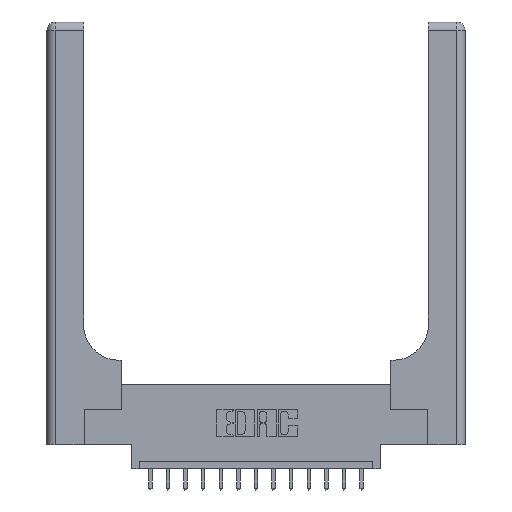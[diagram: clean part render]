
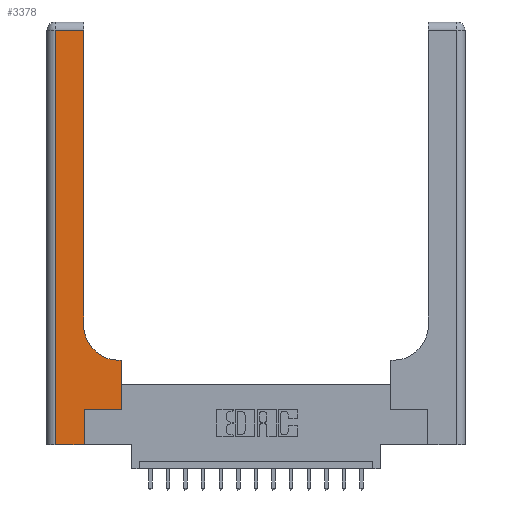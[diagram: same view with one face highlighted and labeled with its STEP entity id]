
A CAD part, top view. The second image highlights one B-rep face of the part: STEP entity #3378.
In plain terms, the highlighted planar face has unit normal (0, 0, 1).
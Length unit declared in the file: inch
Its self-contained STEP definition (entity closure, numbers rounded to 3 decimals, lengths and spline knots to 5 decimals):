
#243 = VECTOR ( 'NONE', #7888, 39.37008 ) ;
#748 = LINE ( 'NONE', #6214, #14005 ) ;
#1354 = VECTOR ( 'NONE', #13960, 39.37008 ) ;
#1579 = PLANE ( 'NONE',  #6849 ) ;
#1590 = VERTEX_POINT ( 'NONE', #4642 ) ;
#1619 = VERTEX_POINT ( 'NONE', #2319 ) ;
#1868 = LINE ( 'NONE', #14319, #16953 ) ;
#1898 = CARTESIAN_POINT ( 'NONE',  ( 0.26, 3., 0.37 ) ) ;
#1962 = CARTESIAN_POINT ( 'NONE',  ( 0.528, 0.6, 0.37 ) ) ;
#2051 = CARTESIAN_POINT ( 'NONE',  ( 0.51, 0.6, 0.37 ) ) ;
#2319 = CARTESIAN_POINT ( 'NONE',  ( 0.528, 0.25, 0.37 ) ) ;
#2332 = ORIENTED_EDGE ( 'NONE', *, *, #17674, .T. ) ;
#2398 = EDGE_CURVE ( 'NONE', #16192, #16802, #6382, .T. ) ;
#2565 = LINE ( 'NONE', #15019, #3959 ) ;
#2573 = DIRECTION ( 'NONE',  ( 1., 0., 0. ) ) ;
#2985 = FACE_OUTER_BOUND ( 'NONE', #3312, .T. ) ;
#3312 = EDGE_LOOP ( 'NONE', ( #5501, #2332, #15300, #16200, #12542, #15239, #9131, #7855, #4134 ) ) ;
#3378 = ADVANCED_FACE ( 'NONE', ( #2985 ), #1579, .F. ) ;
#3959 = VECTOR ( 'NONE', #7848, 39.37008 ) ;
#4134 = ORIENTED_EDGE ( 'NONE', *, *, #4940, .T. ) ;
#4642 = CARTESIAN_POINT ( 'NONE',  ( 0.265, 0., 0.37 ) ) ;
#4940 = EDGE_CURVE ( 'NONE', #8754, #14505, #15435, .T. ) ;
#5501 = ORIENTED_EDGE ( 'NONE', *, *, #15039, .T. ) ;
#6214 = CARTESIAN_POINT ( 'NONE',  ( 0.265, 0.25, 0.37 ) ) ;
#6382 = LINE ( 'NONE', #8626, #243 ) ;
#6792 = CARTESIAN_POINT ( 'NONE',  ( 0.265, 0., 0.37 ) ) ;
#6849 = AXIS2_PLACEMENT_3D ( 'NONE', #14032, #7024, #11344 ) ;
#7024 = DIRECTION ( 'NONE',  ( 0., 0., -1. ) ) ;
#7733 = EDGE_CURVE ( 'NONE', #1619, #10511, #1868, .T. ) ;
#7848 = DIRECTION ( 'NONE',  ( -1., 0., 0. ) ) ;
#7855 = ORIENTED_EDGE ( 'NONE', *, *, #15925, .T. ) ;
#7888 = DIRECTION ( 'NONE',  ( 0., -1., 0. ) ) ;
#8217 = LINE ( 'NONE', #6792, #14340 ) ;
#8593 = VERTEX_POINT ( 'NONE', #10512 ) ;
#8626 = CARTESIAN_POINT ( 'NONE',  ( 0.06, 3., 0.37 ) ) ;
#8656 = CARTESIAN_POINT ( 'NONE',  ( 0.26, 0.6, 0.37 ) ) ;
#8754 = VERTEX_POINT ( 'NONE', #2051 ) ;
#8875 = LINE ( 'NONE', #1898, #11278 ) ;
#9131 = ORIENTED_EDGE ( 'NONE', *, *, #7733, .T. ) ;
#9577 = VERTEX_POINT ( 'NONE', #16522 ) ;
#10511 = VERTEX_POINT ( 'NONE', #1962 ) ;
#10512 = CARTESIAN_POINT ( 'NONE',  ( 0.26, 2.94, 0.37 ) ) ;
#11037 = DIRECTION ( 'NONE',  ( 0., 0., -1. ) ) ;
#11278 = VECTOR ( 'NONE', #11405, 39.37008 ) ;
#11339 = CARTESIAN_POINT ( 'NONE',  ( 0.26, 0.85, 0.37 ) ) ;
#11344 = DIRECTION ( 'NONE',  ( -1., 0., 0. ) ) ;
#11405 = DIRECTION ( 'NONE',  ( 0., 1., 0. ) ) ;
#11468 = DIRECTION ( 'NONE',  ( 0., 1., 0. ) ) ;
#12266 = LINE ( 'NONE', #16285, #13535 ) ;
#12304 = EDGE_CURVE ( 'NONE', #1590, #9577, #8217, .T. ) ;
#12470 = CARTESIAN_POINT ( 'NONE',  ( 0.51, 0.85, 0.37 ) ) ;
#12542 = ORIENTED_EDGE ( 'NONE', *, *, #12304, .T. ) ;
#12650 = EDGE_CURVE ( 'NONE', #16802, #1590, #12266, .T. ) ;
#13535 = VECTOR ( 'NONE', #2573, 39.37008 ) ;
#13960 = DIRECTION ( 'NONE',  ( -1., 0., 0. ) ) ;
#14005 = VECTOR ( 'NONE', #17153, 39.37008 ) ;
#14032 = CARTESIAN_POINT ( 'NONE',  ( 0., 3., 0.37 ) ) ;
#14319 = CARTESIAN_POINT ( 'NONE',  ( 0.528, 0.25, 0.37 ) ) ;
#14340 = VECTOR ( 'NONE', #14526, 39.37008 ) ;
#14505 = VERTEX_POINT ( 'NONE', #11339 ) ;
#14526 = DIRECTION ( 'NONE',  ( 0., 1., 0. ) ) ;
#14557 = AXIS2_PLACEMENT_3D ( 'NONE', #12470, #11037, #15143 ) ;
#14766 = EDGE_CURVE ( 'NONE', #9577, #1619, #748, .T. ) ;
#15019 = CARTESIAN_POINT ( 'NONE',  ( 0., 2.94, 0.37 ) ) ;
#15039 = EDGE_CURVE ( 'NONE', #14505, #8593, #8875, .T. ) ;
#15143 = DIRECTION ( 'NONE',  ( 1., 0., 0. ) ) ;
#15239 = ORIENTED_EDGE ( 'NONE', *, *, #14766, .T. ) ;
#15262 = CARTESIAN_POINT ( 'NONE',  ( 0.06, 0., 0.37 ) ) ;
#15300 = ORIENTED_EDGE ( 'NONE', *, *, #2398, .T. ) ;
#15387 = LINE ( 'NONE', #8656, #1354 ) ;
#15435 = CIRCLE ( 'NONE', #14557, 0.25 ) ;
#15914 = CARTESIAN_POINT ( 'NONE',  ( 0.06, 2.94, 0.37 ) ) ;
#15925 = EDGE_CURVE ( 'NONE', #10511, #8754, #15387, .T. ) ;
#16192 = VERTEX_POINT ( 'NONE', #15914 ) ;
#16200 = ORIENTED_EDGE ( 'NONE', *, *, #12650, .T. ) ;
#16285 = CARTESIAN_POINT ( 'NONE',  ( 0., 0., 0.37 ) ) ;
#16522 = CARTESIAN_POINT ( 'NONE',  ( 0.265, 0.25, 0.37 ) ) ;
#16802 = VERTEX_POINT ( 'NONE', #15262 ) ;
#16953 = VECTOR ( 'NONE', #11468, 39.37008 ) ;
#17153 = DIRECTION ( 'NONE',  ( 1., 0., 0. ) ) ;
#17674 = EDGE_CURVE ( 'NONE', #8593, #16192, #2565, .T. ) ;
